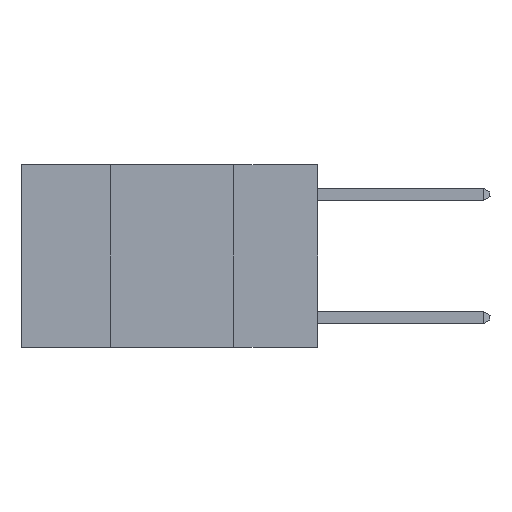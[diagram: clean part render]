
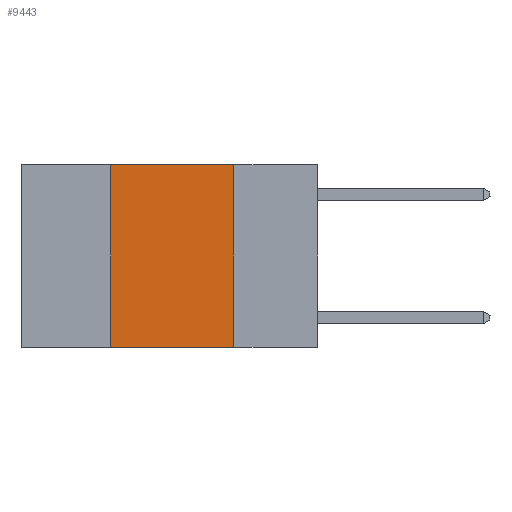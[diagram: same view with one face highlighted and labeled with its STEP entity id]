
A CAD part, left-side view. The second image highlights one B-rep face of the part: STEP entity #9443.
In plain terms, the highlighted planar face has unit normal (-1, 0, 0).
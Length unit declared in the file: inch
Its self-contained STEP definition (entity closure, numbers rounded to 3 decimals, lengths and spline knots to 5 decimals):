
#279 = CARTESIAN_POINT ( 'NONE',  ( 0., 0.17, 0. ) ) ;
#740 = ORIENTED_EDGE ( 'NONE', *, *, #1848, .T. ) ;
#1743 = FACE_OUTER_BOUND ( 'NONE', #14313, .T. ) ;
#1825 = DIRECTION ( 'NONE',  ( 0., -1., 0. ) ) ;
#1848 = EDGE_CURVE ( 'NONE', #19172, #14032, #6373, .T. ) ;
#4733 = EDGE_CURVE ( 'NONE', #19172, #6715, #18224, .T. ) ;
#4752 = LINE ( 'NONE', #14592, #19763 ) ;
#4859 = DIRECTION ( 'NONE',  ( 0., -1., 0. ) ) ;
#4865 = CARTESIAN_POINT ( 'NONE',  ( 0., 0.42, 0. ) ) ;
#4974 = DIRECTION ( 'NONE',  ( 0., 0., 1. ) ) ;
#5133 = VECTOR ( 'NONE', #4859, 39.37008 ) ;
#5494 = EDGE_CURVE ( 'NONE', #15968, #14032, #12504, .T. ) ;
#6373 = LINE ( 'NONE', #9841, #5133 ) ;
#6715 = VERTEX_POINT ( 'NONE', #14546 ) ;
#7979 = PLANE ( 'NONE',  #20619 ) ;
#9225 = CARTESIAN_POINT ( 'NONE',  ( 0., 0.17, -0.37 ) ) ;
#9443 = ADVANCED_FACE ( 'NONE', ( #1743 ), #7979, .F. ) ;
#9841 = CARTESIAN_POINT ( 'NONE',  ( 0., 0.6, -0.37 ) ) ;
#10163 = ORIENTED_EDGE ( 'NONE', *, *, #15110, .F. ) ;
#11217 = DIRECTION ( 'NONE',  ( 0., 0., -1. ) ) ;
#11254 = ORIENTED_EDGE ( 'NONE', *, *, #4733, .F. ) ;
#11315 = VECTOR ( 'NONE', #4974, 39.37008 ) ;
#12504 = LINE ( 'NONE', #20789, #17424 ) ;
#13107 = CARTESIAN_POINT ( 'NONE',  ( 0., 0.42, -0.37 ) ) ;
#14032 = VERTEX_POINT ( 'NONE', #9225 ) ;
#14313 = EDGE_LOOP ( 'NONE', ( #19678, #10163, #11254, #740 ) ) ;
#14546 = CARTESIAN_POINT ( 'NONE',  ( 0., 0.42, 0. ) ) ;
#14582 = DIRECTION ( 'NONE',  ( 0., 0., -1. ) ) ;
#14592 = CARTESIAN_POINT ( 'NONE',  ( 0., 0.6, 0. ) ) ;
#15110 = EDGE_CURVE ( 'NONE', #6715, #15968, #4752, .T. ) ;
#15968 = VERTEX_POINT ( 'NONE', #279 ) ;
#17424 = VECTOR ( 'NONE', #11217, 39.37008 ) ;
#18224 = LINE ( 'NONE', #4865, #11315 ) ;
#19172 = VERTEX_POINT ( 'NONE', #13107 ) ;
#19407 = DIRECTION ( 'NONE',  ( 1., 0., 0. ) ) ;
#19510 = CARTESIAN_POINT ( 'NONE',  ( 0., 0.6, 0. ) ) ;
#19678 = ORIENTED_EDGE ( 'NONE', *, *, #5494, .F. ) ;
#19763 = VECTOR ( 'NONE', #1825, 39.37008 ) ;
#20619 = AXIS2_PLACEMENT_3D ( 'NONE', #19510, #19407, #14582 ) ;
#20789 = CARTESIAN_POINT ( 'NONE',  ( 0., 0.17, 0. ) ) ;
